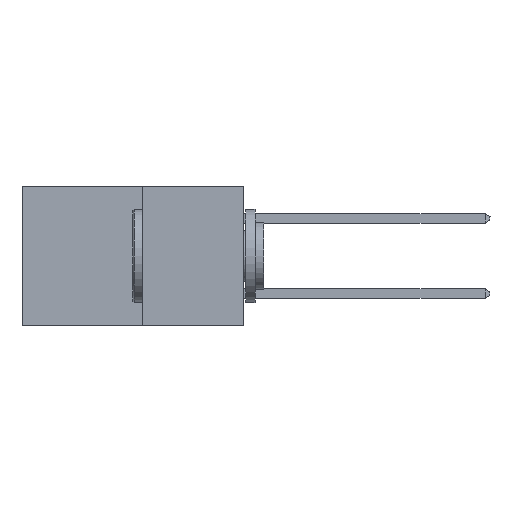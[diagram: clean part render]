
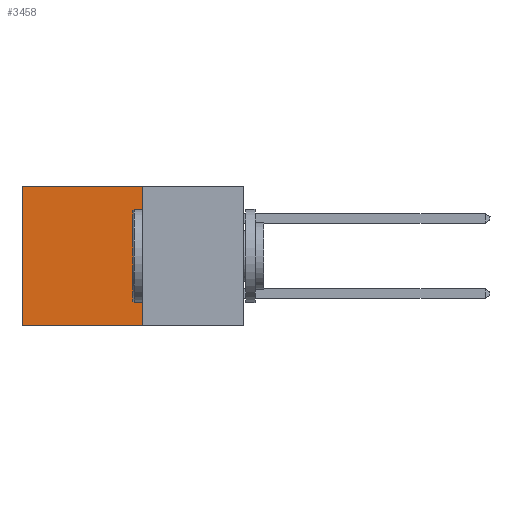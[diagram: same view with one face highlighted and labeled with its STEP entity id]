
A CAD part, left-side view. The second image highlights one B-rep face of the part: STEP entity #3458.
In plain terms, the highlighted planar face has unit normal (-1, 0, 0).
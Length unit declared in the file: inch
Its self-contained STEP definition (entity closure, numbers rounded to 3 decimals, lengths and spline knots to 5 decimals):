
#733 = VERTEX_POINT ( 'NONE', #8941 ) ;
#2005 = AXIS2_PLACEMENT_3D ( 'NONE', #17811, #17721, #17613 ) ;
#2043 = EDGE_CURVE ( 'NONE', #19739, #16266, #20501, .T. ) ;
#2552 = LINE ( 'NONE', #23188, #7395 ) ;
#2984 = ORIENTED_EDGE ( 'NONE', *, *, #26304, .T. ) ;
#3458 = ADVANCED_FACE ( 'NONE', ( #8613 ), #19653, .F. ) ;
#3706 = VECTOR ( 'NONE', #13487, 39.37008 ) ;
#5265 = CARTESIAN_POINT ( 'NONE',  ( 0.277, 0.27, -0.37 ) ) ;
#5649 = EDGE_LOOP ( 'NONE', ( #12698, #18155, #23564, #2984 ) ) ;
#5739 = CARTESIAN_POINT ( 'NONE',  ( 0.277, 0.27, -0.37 ) ) ;
#5819 = CARTESIAN_POINT ( 'NONE',  ( 0.277, 0.27, 0. ) ) ;
#7395 = VECTOR ( 'NONE', #19091, 39.37008 ) ;
#8007 = EDGE_CURVE ( 'NONE', #16266, #12290, #17978, .T. ) ;
#8613 = FACE_OUTER_BOUND ( 'NONE', #5649, .T. ) ;
#8941 = CARTESIAN_POINT ( 'NONE',  ( 0.277, 0.59, 0. ) ) ;
#10030 = CARTESIAN_POINT ( 'NONE',  ( 0.277, 0.59, -0.37 ) ) ;
#11394 = CARTESIAN_POINT ( 'NONE',  ( 0.277, 0.59, -0.37 ) ) ;
#12100 = CARTESIAN_POINT ( 'NONE',  ( 0.277, 0.27, -0.37 ) ) ;
#12290 = VERTEX_POINT ( 'NONE', #10030 ) ;
#12698 = ORIENTED_EDGE ( 'NONE', *, *, #18753, .T. ) ;
#13487 = DIRECTION ( 'NONE',  ( 0., 0., -1. ) ) ;
#14470 = VECTOR ( 'NONE', #22172, 39.37008 ) ;
#16266 = VERTEX_POINT ( 'NONE', #5265 ) ;
#17613 = DIRECTION ( 'NONE',  ( 0., 0., -1. ) ) ;
#17721 = DIRECTION ( 'NONE',  ( 1., 0., 0. ) ) ;
#17811 = CARTESIAN_POINT ( 'NONE',  ( 0.277, 0.27, -0.37 ) ) ;
#17978 = LINE ( 'NONE', #12100, #22731 ) ;
#18155 = ORIENTED_EDGE ( 'NONE', *, *, #8007, .F. ) ;
#18753 = EDGE_CURVE ( 'NONE', #733, #12290, #20110, .T. ) ;
#19091 = DIRECTION ( 'NONE',  ( 0., 1., 0. ) ) ;
#19653 = PLANE ( 'NONE',  #2005 ) ;
#19739 = VERTEX_POINT ( 'NONE', #5819 ) ;
#20110 = LINE ( 'NONE', #11394, #3706 ) ;
#20293 = DIRECTION ( 'NONE',  ( 0., 1., 0. ) ) ;
#20501 = LINE ( 'NONE', #5739, #14470 ) ;
#22172 = DIRECTION ( 'NONE',  ( 0., 0., -1. ) ) ;
#22731 = VECTOR ( 'NONE', #20293, 39.37008 ) ;
#23188 = CARTESIAN_POINT ( 'NONE',  ( 0.277, 0.27, 0. ) ) ;
#23564 = ORIENTED_EDGE ( 'NONE', *, *, #2043, .F. ) ;
#26304 = EDGE_CURVE ( 'NONE', #19739, #733, #2552, .T. ) ;
